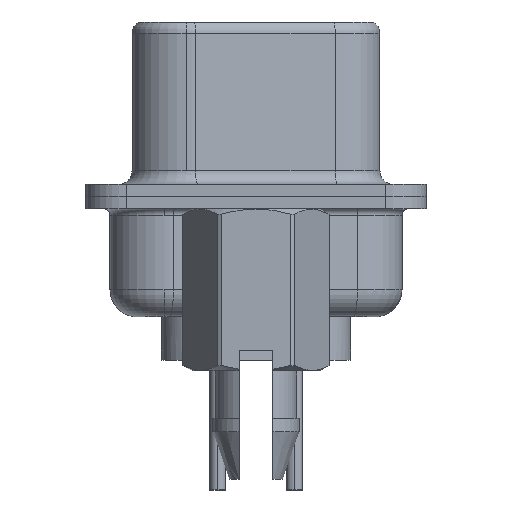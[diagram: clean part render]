
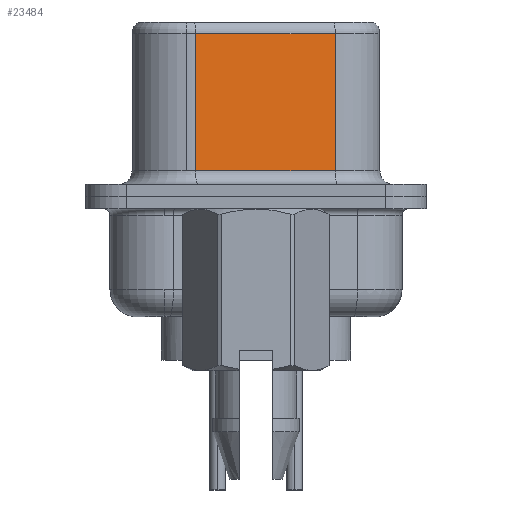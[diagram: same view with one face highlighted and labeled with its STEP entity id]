
A CAD part, left-side view. The second image highlights one B-rep face of the part: STEP entity #23484.
In plain terms, the highlighted planar face has unit normal (-0.985, -0.174, 0).
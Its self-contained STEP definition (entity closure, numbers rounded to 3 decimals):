
#177 = ORIENTED_EDGE ( 'NONE', *, *, #12565, .T. ) ;
#805 = LINE ( 'NONE', #2404, #5200 ) ;
#832 = LINE ( 'NONE', #6799, #24358 ) ;
#1213 = CARTESIAN_POINT ( 'NONE',  ( 4.58, -2.927, 0.95 ) ) ;
#2404 = CARTESIAN_POINT ( 'NONE',  ( 4.58, -2.927, 6.02 ) ) ;
#3201 = LINE ( 'NONE', #1213, #12844 ) ;
#3313 = ORIENTED_EDGE ( 'NONE', *, *, #14092, .T. ) ;
#3554 = ORIENTED_EDGE ( 'NONE', *, *, #19367, .F. ) ;
#3746 = CARTESIAN_POINT ( 'NONE',  ( 4.58, -2.927, 0.95 ) ) ;
#4282 = VERTEX_POINT ( 'NONE', #17143 ) ;
#4777 = VERTEX_POINT ( 'NONE', #7130 ) ;
#5200 = VECTOR ( 'NONE', #8893, 1000. ) ;
#6799 = CARTESIAN_POINT ( 'NONE',  ( 3.67, 2.233, 6.52 ) ) ;
#7130 = CARTESIAN_POINT ( 'NONE',  ( 4.58, -2.927, 6.02 ) ) ;
#8258 = CARTESIAN_POINT ( 'NONE',  ( 4.58, -2.927, 6.52 ) ) ;
#8451 = PLANE ( 'NONE',  #8676 ) ;
#8676 = AXIS2_PLACEMENT_3D ( 'NONE', #12957, #10962, #16542 ) ;
#8893 = DIRECTION ( 'NONE',  ( -0.174, 0.985, 0. ) ) ;
#9711 = VERTEX_POINT ( 'NONE', #3746 ) ;
#10962 = DIRECTION ( 'NONE',  ( 0.985, 0.174, 0. ) ) ;
#11679 = CARTESIAN_POINT ( 'NONE',  ( 3.67, 2.233, 6.02 ) ) ;
#12240 = LINE ( 'NONE', #8258, #19621 ) ;
#12319 = EDGE_LOOP ( 'NONE', ( #3554, #177, #20362, #3313 ) ) ;
#12565 = EDGE_CURVE ( 'NONE', #4777, #22612, #805, .T. ) ;
#12844 = VECTOR ( 'NONE', #23545, 1000. ) ;
#12957 = CARTESIAN_POINT ( 'NONE',  ( 4.58, -2.927, 6.52 ) ) ;
#14092 = EDGE_CURVE ( 'NONE', #4282, #9711, #3201, .T. ) ;
#14738 = EDGE_CURVE ( 'NONE', #22612, #4282, #832, .T. ) ;
#14905 = DIRECTION ( 'NONE',  ( 0., 0., -1. ) ) ;
#16352 = DIRECTION ( 'NONE',  ( 0., 0., -1. ) ) ;
#16542 = DIRECTION ( 'NONE',  ( -0.174, 0.985, 0. ) ) ;
#17143 = CARTESIAN_POINT ( 'NONE',  ( 3.67, 2.233, 0.95 ) ) ;
#19367 = EDGE_CURVE ( 'NONE', #4777, #9711, #12240, .T. ) ;
#19621 = VECTOR ( 'NONE', #16352, 1000. ) ;
#20362 = ORIENTED_EDGE ( 'NONE', *, *, #14738, .T. ) ;
#22612 = VERTEX_POINT ( 'NONE', #11679 ) ;
#23484 = ADVANCED_FACE ( 'NONE', ( #25098 ), #8451, .F. ) ;
#23545 = DIRECTION ( 'NONE',  ( 0.174, -0.985, 0. ) ) ;
#24358 = VECTOR ( 'NONE', #14905, 1000. ) ;
#25098 = FACE_OUTER_BOUND ( 'NONE', #12319, .T. ) ;
